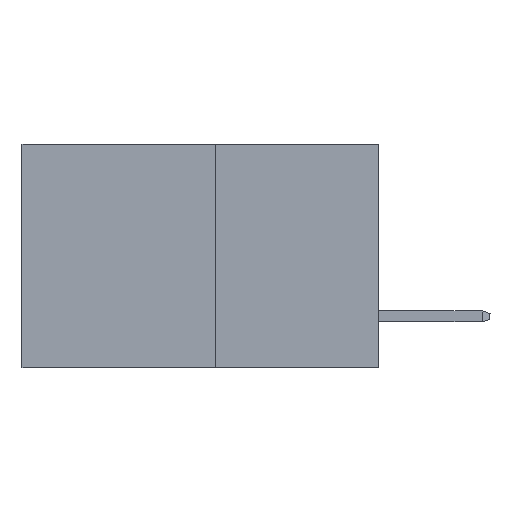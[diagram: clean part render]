
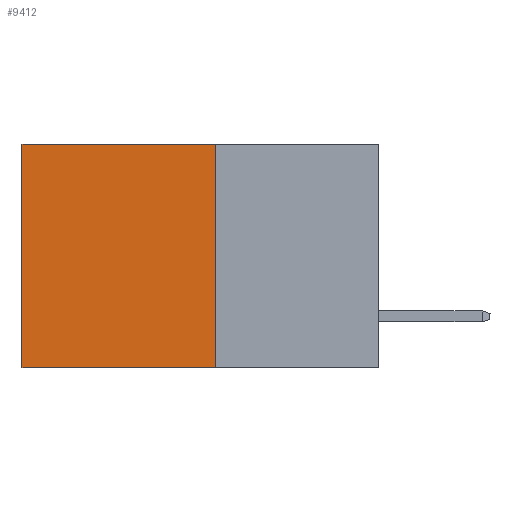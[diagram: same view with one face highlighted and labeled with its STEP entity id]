
A CAD part, left-side view. The second image highlights one B-rep face of the part: STEP entity #9412.
In plain terms, the highlighted planar face has unit normal (-1, 0, 0).
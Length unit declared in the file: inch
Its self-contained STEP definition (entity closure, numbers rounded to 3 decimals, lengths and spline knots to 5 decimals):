
#413 = EDGE_CURVE ( 'NONE', #3415, #9355, #6529, .T. ) ;
#1011 = VECTOR ( 'NONE', #2301, 39.37008 ) ;
#1302 = EDGE_LOOP ( 'NONE', ( #3070, #9280, #7132, #5000 ) ) ;
#2191 = VECTOR ( 'NONE', #8673, 39.37008 ) ;
#2301 = DIRECTION ( 'NONE',  ( 0., 1., 0. ) ) ;
#2421 = CARTESIAN_POINT ( 'NONE',  ( 0.277, 0.27, 0. ) ) ;
#2471 = VERTEX_POINT ( 'NONE', #9856 ) ;
#2850 = EDGE_CURVE ( 'NONE', #5358, #3415, #3959, .T. ) ;
#2919 = CARTESIAN_POINT ( 'NONE',  ( 0.277, 0.27, -0.37 ) ) ;
#3070 = ORIENTED_EDGE ( 'NONE', *, *, #7170, .T. ) ;
#3415 = VERTEX_POINT ( 'NONE', #5069 ) ;
#3886 = DIRECTION ( 'NONE',  ( 0., 0., -1. ) ) ;
#3959 = LINE ( 'NONE', #2919, #10119 ) ;
#3970 = FACE_OUTER_BOUND ( 'NONE', #1302, .T. ) ;
#5000 = ORIENTED_EDGE ( 'NONE', *, *, #7598, .T. ) ;
#5069 = CARTESIAN_POINT ( 'NONE',  ( 0.277, 0.27, -0.37 ) ) ;
#5306 = VECTOR ( 'NONE', #5741, 39.37008 ) ;
#5358 = VERTEX_POINT ( 'NONE', #9718 ) ;
#5558 = DIRECTION ( 'NONE',  ( 0., 0., -1. ) ) ;
#5569 = DIRECTION ( 'NONE',  ( 1., 0., 0. ) ) ;
#5693 = CARTESIAN_POINT ( 'NONE',  ( 0.277, 0.27, -0.37 ) ) ;
#5741 = DIRECTION ( 'NONE',  ( 0., 0., -1. ) ) ;
#5832 = PLANE ( 'NONE',  #9766 ) ;
#6242 = CARTESIAN_POINT ( 'NONE',  ( 0.277, 0.59, -0.37 ) ) ;
#6529 = LINE ( 'NONE', #10203, #2191 ) ;
#7132 = ORIENTED_EDGE ( 'NONE', *, *, #2850, .F. ) ;
#7170 = EDGE_CURVE ( 'NONE', #2471, #9355, #9595, .T. ) ;
#7595 = LINE ( 'NONE', #2421, #1011 ) ;
#7598 = EDGE_CURVE ( 'NONE', #5358, #2471, #7595, .T. ) ;
#8565 = CARTESIAN_POINT ( 'NONE',  ( 0.277, 0.59, -0.37 ) ) ;
#8673 = DIRECTION ( 'NONE',  ( 0., 1., 0. ) ) ;
#9280 = ORIENTED_EDGE ( 'NONE', *, *, #413, .F. ) ;
#9355 = VERTEX_POINT ( 'NONE', #6242 ) ;
#9412 = ADVANCED_FACE ( 'NONE', ( #3970 ), #5832, .F. ) ;
#9595 = LINE ( 'NONE', #8565, #5306 ) ;
#9718 = CARTESIAN_POINT ( 'NONE',  ( 0.277, 0.27, 0. ) ) ;
#9766 = AXIS2_PLACEMENT_3D ( 'NONE', #5693, #5569, #5558 ) ;
#9856 = CARTESIAN_POINT ( 'NONE',  ( 0.277, 0.59, 0. ) ) ;
#10119 = VECTOR ( 'NONE', #3886, 39.37008 ) ;
#10203 = CARTESIAN_POINT ( 'NONE',  ( 0.277, 0.27, -0.37 ) ) ;
